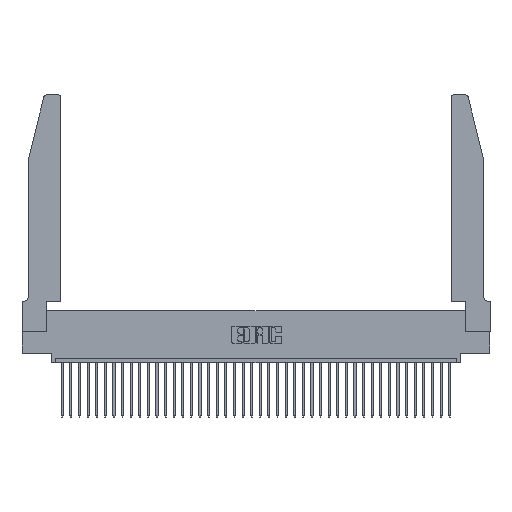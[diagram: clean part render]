
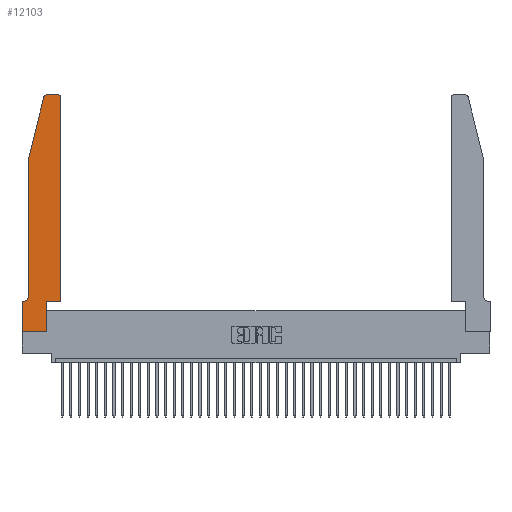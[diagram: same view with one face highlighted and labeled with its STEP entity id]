
A CAD part, top view. The second image highlights one B-rep face of the part: STEP entity #12103.
In plain terms, the highlighted planar face has unit normal (0, 0, 1).
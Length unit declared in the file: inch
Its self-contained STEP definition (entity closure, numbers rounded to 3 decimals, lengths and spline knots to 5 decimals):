
#51 = VECTOR ( 'NONE', #5577, 39.37008 ) ;
#513 = CARTESIAN_POINT ( 'NONE',  ( 0.0755, 2., 0.37 ) ) ;
#1283 = VERTEX_POINT ( 'NONE', #22424 ) ;
#1629 = DIRECTION ( 'NONE',  ( 1., 0., 0. ) ) ;
#1763 = DIRECTION ( 'NONE',  ( -1., 0., 0. ) ) ;
#1770 = CARTESIAN_POINT ( 'NONE',  ( 0.2605, 2.75, 0.37 ) ) ;
#1925 = LINE ( 'NONE', #6238, #9947 ) ;
#2174 = ORIENTED_EDGE ( 'NONE', *, *, #7428, .T. ) ;
#3329 = LINE ( 'NONE', #31290, #16146 ) ;
#3645 = VERTEX_POINT ( 'NONE', #37889 ) ;
#4297 = LINE ( 'NONE', #1770, #51 ) ;
#4493 = CARTESIAN_POINT ( 'NONE',  ( 0.4505, 0.35, 0.37 ) ) ;
#4775 = CIRCLE ( 'NONE', #37027, 0.03 ) ;
#5329 = VERTEX_POINT ( 'NONE', #24396 ) ;
#5577 = DIRECTION ( 'NONE',  ( -1., 0., 0. ) ) ;
#5789 = VECTOR ( 'NONE', #1763, 39.37008 ) ;
#6115 = CIRCLE ( 'NONE', #28896, 0.03 ) ;
#6238 = CARTESIAN_POINT ( 'NONE',  ( 0., 0., 0.37 ) ) ;
#6246 = CARTESIAN_POINT ( 'NONE',  ( 0.4505, 2.72, 0.37 ) ) ;
#7428 = EDGE_CURVE ( 'NONE', #5329, #20288, #26667, .T. ) ;
#7900 = VERTEX_POINT ( 'NONE', #4493 ) ;
#8016 = CARTESIAN_POINT ( 'NONE',  ( 0.4505, 0.35, 0.37 ) ) ;
#8093 = ORIENTED_EDGE ( 'NONE', *, *, #22775, .T. ) ;
#9247 = VECTOR ( 'NONE', #16159, 39.37008 ) ;
#9947 = VECTOR ( 'NONE', #30471, 39.37008 ) ;
#10057 = DIRECTION ( 'NONE',  ( 0., -1., 0. ) ) ;
#10216 = CARTESIAN_POINT ( 'NONE',  ( 0.0055, 0.42, 0.37 ) ) ;
#10405 = CARTESIAN_POINT ( 'NONE',  ( 0.4205, 2.75, 0.37 ) ) ;
#10786 = CARTESIAN_POINT ( 'NONE',  ( 0.2865, 0.35, 0.37 ) ) ;
#10864 = VERTEX_POINT ( 'NONE', #10405 ) ;
#10952 = DIRECTION ( 'NONE',  ( 0., 1., 0. ) ) ;
#11278 = CARTESIAN_POINT ( 'NONE',  ( 0.25487, 2.72718, 0.37 ) ) ;
#11289 = ORIENTED_EDGE ( 'NONE', *, *, #34127, .T. ) ;
#11746 = VECTOR ( 'NONE', #10057, 39.37008 ) ;
#11931 = EDGE_CURVE ( 'NONE', #27161, #5329, #31525, .T. ) ;
#12032 = ORIENTED_EDGE ( 'NONE', *, *, #20662, .T. ) ;
#12103 = ADVANCED_FACE ( 'NONE', ( #27258 ), #29375, .T. ) ;
#13130 = EDGE_LOOP ( 'NONE', ( #35622, #23349, #14598, #32684, #2174, #22908, #28249, #26175, #8093, #12032, #11289, #24002 ) ) ;
#13246 = DIRECTION ( 'NONE',  ( 1., 0., 0. ) ) ;
#13881 = DIRECTION ( 'NONE',  ( 1., 0., 0. ) ) ;
#14566 = LINE ( 'NONE', #20217, #28676 ) ;
#14598 = ORIENTED_EDGE ( 'NONE', *, *, #28101, .T. ) ;
#15214 = AXIS2_PLACEMENT_3D ( 'NONE', #35014, #37772, #35772 ) ;
#16146 = VECTOR ( 'NONE', #1629, 39.37008 ) ;
#16159 = DIRECTION ( 'NONE',  ( 0., -1., 0. ) ) ;
#16260 = EDGE_CURVE ( 'NONE', #10864, #1283, #4297, .T. ) ;
#16852 = CARTESIAN_POINT ( 'NONE',  ( 0.2865, 0., 0.37 ) ) ;
#17150 = EDGE_CURVE ( 'NONE', #3645, #35186, #30444, .T. ) ;
#18797 = VERTEX_POINT ( 'NONE', #16852 ) ;
#19074 = EDGE_CURVE ( 'NONE', #20288, #3645, #21827, .T. ) ;
#20217 = CARTESIAN_POINT ( 'NONE',  ( 0.0755, 2., 0.37 ) ) ;
#20228 = EDGE_CURVE ( 'NONE', #35186, #18797, #1925, .T. ) ;
#20288 = VERTEX_POINT ( 'NONE', #34798 ) ;
#20314 = VECTOR ( 'NONE', #10952, 39.37008 ) ;
#20662 = EDGE_CURVE ( 'NONE', #33989, #7900, #3329, .T. ) ;
#20887 = EDGE_CURVE ( 'NONE', #34421, #10864, #4775, .T. ) ;
#21628 = CARTESIAN_POINT ( 'NONE',  ( 0., 0., 0.37 ) ) ;
#21827 = LINE ( 'NONE', #22749, #5789 ) ;
#22424 = CARTESIAN_POINT ( 'NONE',  ( 0.284, 2.75, 0.37 ) ) ;
#22749 = CARTESIAN_POINT ( 'NONE',  ( 0.0755, 0.35, 0.37 ) ) ;
#22774 = VERTEX_POINT ( 'NONE', #11278 ) ;
#22775 = EDGE_CURVE ( 'NONE', #18797, #33989, #26203, .T. ) ;
#22908 = ORIENTED_EDGE ( 'NONE', *, *, #19074, .T. ) ;
#23267 = AXIS2_PLACEMENT_3D ( 'NONE', #10216, #31271, #28513 ) ;
#23349 = ORIENTED_EDGE ( 'NONE', *, *, #25852, .T. ) ;
#24002 = ORIENTED_EDGE ( 'NONE', *, *, #20887, .T. ) ;
#24396 = CARTESIAN_POINT ( 'NONE',  ( 0.0755, 0.42, 0.37 ) ) ;
#25073 = CARTESIAN_POINT ( 'NONE',  ( 0., 0., 0.37 ) ) ;
#25807 = CARTESIAN_POINT ( 'NONE',  ( 0.284, 2.72, 0.37 ) ) ;
#25852 = EDGE_CURVE ( 'NONE', #1283, #22774, #6115, .T. ) ;
#25941 = DIRECTION ( 'NONE',  ( 0., 0., 1. ) ) ;
#26128 = DIRECTION ( 'NONE',  ( 0., 1., 0. ) ) ;
#26175 = ORIENTED_EDGE ( 'NONE', *, *, #20228, .T. ) ;
#26203 = LINE ( 'NONE', #26393, #31381 ) ;
#26393 = CARTESIAN_POINT ( 'NONE',  ( 0.2865, 0.35, 0.37 ) ) ;
#26667 = CIRCLE ( 'NONE', #23267, 0.07 ) ;
#26853 = LINE ( 'NONE', #8016, #20314 ) ;
#27161 = VERTEX_POINT ( 'NONE', #513 ) ;
#27258 = FACE_OUTER_BOUND ( 'NONE', #13130, .T. ) ;
#28101 = EDGE_CURVE ( 'NONE', #22774, #27161, #14566, .T. ) ;
#28249 = ORIENTED_EDGE ( 'NONE', *, *, #17150, .T. ) ;
#28513 = DIRECTION ( 'NONE',  ( -1., 0., 0. ) ) ;
#28676 = VECTOR ( 'NONE', #35309, 39.37008 ) ;
#28896 = AXIS2_PLACEMENT_3D ( 'NONE', #25807, #25941, #13881 ) ;
#29375 = PLANE ( 'NONE',  #15214 ) ;
#30444 = LINE ( 'NONE', #25073, #9247 ) ;
#30471 = DIRECTION ( 'NONE',  ( 1., 0., 0. ) ) ;
#30545 = CARTESIAN_POINT ( 'NONE',  ( 0.4205, 2.72, 0.37 ) ) ;
#31271 = DIRECTION ( 'NONE',  ( 0., 0., -1. ) ) ;
#31290 = CARTESIAN_POINT ( 'NONE',  ( 0.4505, 0.35, 0.37 ) ) ;
#31381 = VECTOR ( 'NONE', #26128, 39.37008 ) ;
#31525 = LINE ( 'NONE', #37405, #11746 ) ;
#32684 = ORIENTED_EDGE ( 'NONE', *, *, #11931, .T. ) ;
#33989 = VERTEX_POINT ( 'NONE', #10786 ) ;
#34127 = EDGE_CURVE ( 'NONE', #7900, #34421, #26853, .T. ) ;
#34421 = VERTEX_POINT ( 'NONE', #6246 ) ;
#34798 = CARTESIAN_POINT ( 'NONE',  ( 0.0055, 0.35, 0.37 ) ) ;
#35014 = CARTESIAN_POINT ( 'NONE',  ( 0., 0.35, 0.37 ) ) ;
#35186 = VERTEX_POINT ( 'NONE', #21628 ) ;
#35309 = DIRECTION ( 'NONE',  ( -0.239, -0.971, 0. ) ) ;
#35622 = ORIENTED_EDGE ( 'NONE', *, *, #16260, .T. ) ;
#35772 = DIRECTION ( 'NONE',  ( 1., 0., 0. ) ) ;
#36723 = DIRECTION ( 'NONE',  ( 0., 0., 1. ) ) ;
#37027 = AXIS2_PLACEMENT_3D ( 'NONE', #30545, #36723, #13246 ) ;
#37405 = CARTESIAN_POINT ( 'NONE',  ( 0.0755, 2., 0.37 ) ) ;
#37772 = DIRECTION ( 'NONE',  ( 0., 0., 1. ) ) ;
#37889 = CARTESIAN_POINT ( 'NONE',  ( 0., 0.35, 0.37 ) ) ;
